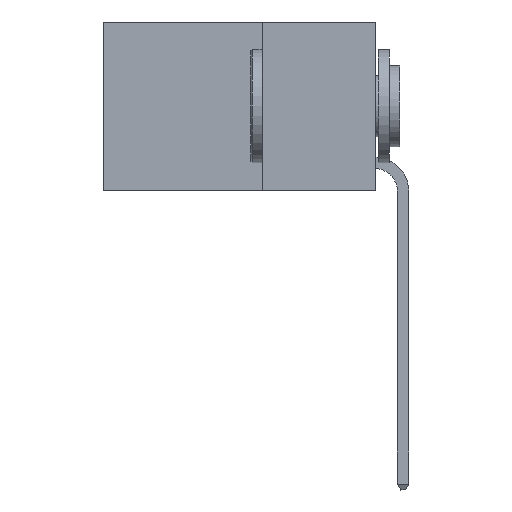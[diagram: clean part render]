
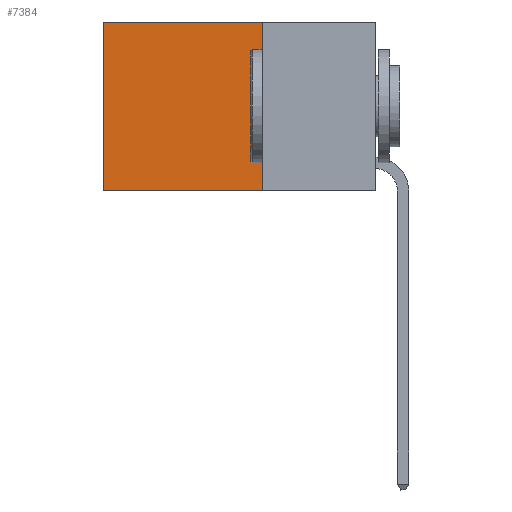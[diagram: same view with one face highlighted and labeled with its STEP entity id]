
A CAD part, left-side view. The second image highlights one B-rep face of the part: STEP entity #7384.
In plain terms, the highlighted planar face has unit normal (-1, 0, 0).
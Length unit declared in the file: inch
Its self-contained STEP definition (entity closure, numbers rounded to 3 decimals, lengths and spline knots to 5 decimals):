
#448 = DIRECTION ( 'NONE',  ( 0., 1., 0. ) ) ;
#1342 = DIRECTION ( 'NONE',  ( 0., 0., -1. ) ) ;
#1510 = EDGE_CURVE ( 'NONE', #7920, #5772, #3130, .T. ) ;
#1660 = ORIENTED_EDGE ( 'NONE', *, *, #8524, .T. ) ;
#2131 = LINE ( 'NONE', #2193, #3762 ) ;
#2193 = CARTESIAN_POINT ( 'NONE',  ( 0.2625, 0.6, 0. ) ) ;
#2251 = LINE ( 'NONE', #6032, #12156 ) ;
#2666 = EDGE_LOOP ( 'NONE', ( #1660, #12100, #4535, #8854 ) ) ;
#2674 = PLANE ( 'NONE',  #9063 ) ;
#3130 = LINE ( 'NONE', #10650, #5528 ) ;
#3242 = VERTEX_POINT ( 'NONE', #7735 ) ;
#3762 = VECTOR ( 'NONE', #11727, 39.37008 ) ;
#4124 = EDGE_CURVE ( 'NONE', #3242, #8983, #6919, .T. ) ;
#4535 = ORIENTED_EDGE ( 'NONE', *, *, #4875, .F. ) ;
#4875 = EDGE_CURVE ( 'NONE', #7920, #3242, #2251, .T. ) ;
#5218 = DIRECTION ( 'NONE',  ( 0., 1., 0. ) ) ;
#5528 = VECTOR ( 'NONE', #5218, 39.37008 ) ;
#5651 = FACE_OUTER_BOUND ( 'NONE', #2666, .T. ) ;
#5655 = VECTOR ( 'NONE', #448, 39.37008 ) ;
#5772 = VERTEX_POINT ( 'NONE', #11796 ) ;
#6032 = CARTESIAN_POINT ( 'NONE',  ( 0.2625, 0.25, 0. ) ) ;
#6919 = LINE ( 'NONE', #10666, #5655 ) ;
#7384 = ADVANCED_FACE ( 'NONE', ( #5651 ), #2674, .F. ) ;
#7735 = CARTESIAN_POINT ( 'NONE',  ( 0.2625, 0.25, -0.37 ) ) ;
#7920 = VERTEX_POINT ( 'NONE', #11275 ) ;
#8524 = EDGE_CURVE ( 'NONE', #5772, #8983, #2131, .T. ) ;
#8854 = ORIENTED_EDGE ( 'NONE', *, *, #1510, .T. ) ;
#8983 = VERTEX_POINT ( 'NONE', #9108 ) ;
#9063 = AXIS2_PLACEMENT_3D ( 'NONE', #10258, #11052, #12150 ) ;
#9108 = CARTESIAN_POINT ( 'NONE',  ( 0.2625, 0.6, -0.37 ) ) ;
#10258 = CARTESIAN_POINT ( 'NONE',  ( 0.2625, 0.25, 0. ) ) ;
#10650 = CARTESIAN_POINT ( 'NONE',  ( 0.2625, 0.25, 0. ) ) ;
#10666 = CARTESIAN_POINT ( 'NONE',  ( 0.2625, 0.25, -0.37 ) ) ;
#11052 = DIRECTION ( 'NONE',  ( 1., 0., 0. ) ) ;
#11275 = CARTESIAN_POINT ( 'NONE',  ( 0.2625, 0.25, 0. ) ) ;
#11727 = DIRECTION ( 'NONE',  ( 0., 0., -1. ) ) ;
#11796 = CARTESIAN_POINT ( 'NONE',  ( 0.2625, 0.6, 0. ) ) ;
#12100 = ORIENTED_EDGE ( 'NONE', *, *, #4124, .F. ) ;
#12150 = DIRECTION ( 'NONE',  ( 0., 0., -1. ) ) ;
#12156 = VECTOR ( 'NONE', #1342, 39.37008 ) ;
